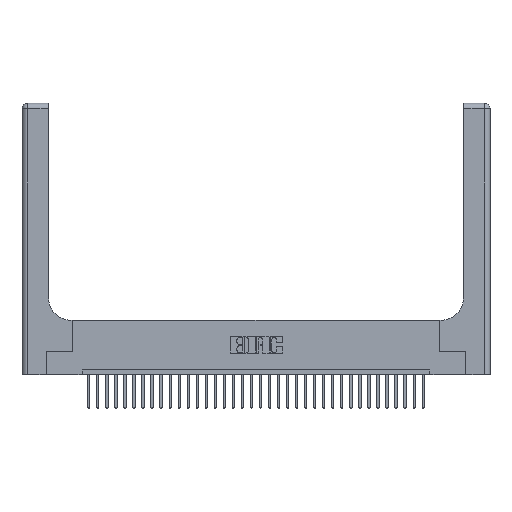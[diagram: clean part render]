
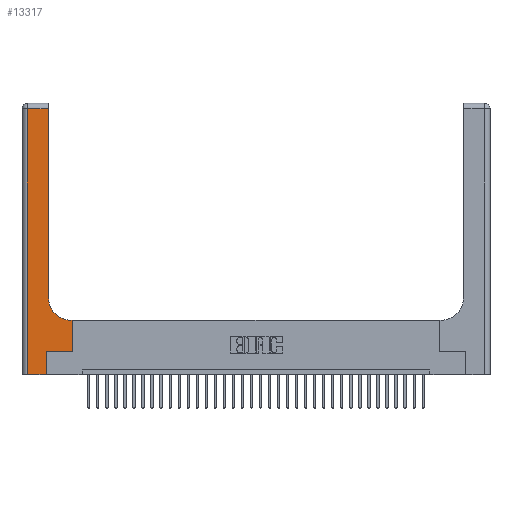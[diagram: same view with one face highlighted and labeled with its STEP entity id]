
A CAD part, top view. The second image highlights one B-rep face of the part: STEP entity #13317.
In plain terms, the highlighted planar face has unit normal (0, 0, 1).
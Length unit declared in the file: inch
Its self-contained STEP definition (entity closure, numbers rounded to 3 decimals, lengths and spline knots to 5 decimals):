
#956 = CARTESIAN_POINT ( 'NONE',  ( 0.5415, 0.6, 0.37 ) ) ;
#1182 = CARTESIAN_POINT ( 'NONE',  ( 0.06, 2.94, 0.37 ) ) ;
#1258 = EDGE_CURVE ( 'NONE', #16805, #28091, #2819, .T. ) ;
#2010 = ORIENTED_EDGE ( 'NONE', *, *, #9235, .T. ) ;
#2102 = CARTESIAN_POINT ( 'NONE',  ( 0.2915, 0.6, 0.37 ) ) ;
#2819 = LINE ( 'NONE', #2102, #31387 ) ;
#2953 = VERTEX_POINT ( 'NONE', #7476 ) ;
#4303 = DIRECTION ( 'NONE',  ( 0., 1., 0. ) ) ;
#4928 = LINE ( 'NONE', #17188, #25613 ) ;
#5272 = LINE ( 'NONE', #17561, #27623 ) ;
#5859 = LINE ( 'NONE', #9953, #17491 ) ;
#6303 = ORIENTED_EDGE ( 'NONE', *, *, #15693, .T. ) ;
#6751 = CARTESIAN_POINT ( 'NONE',  ( 0., 3., 0.37 ) ) ;
#7102 = DIRECTION ( 'NONE',  ( 0., 0., -1. ) ) ;
#7476 = CARTESIAN_POINT ( 'NONE',  ( 0.2915, 0.85, 0.37 ) ) ;
#7660 = CIRCLE ( 'NONE', #20442, 0.25 ) ;
#8048 = VECTOR ( 'NONE', #4303, 39.37008 ) ;
#8104 = EDGE_LOOP ( 'NONE', ( #2010, #31231, #11013, #26593, #19111, #23381, #6303, #32745, #13252 ) ) ;
#8787 = DIRECTION ( 'NONE',  ( 0., -1., 0. ) ) ;
#9042 = VECTOR ( 'NONE', #18088, 39.37008 ) ;
#9235 = EDGE_CURVE ( 'NONE', #2953, #24137, #32086, .T. ) ;
#9812 = LINE ( 'NONE', #19472, #18540 ) ;
#9953 = CARTESIAN_POINT ( 'NONE',  ( 0., 0., 0.37 ) ) ;
#10072 = CARTESIAN_POINT ( 'NONE',  ( 0.269, 0., 0.37 ) ) ;
#10834 = EDGE_CURVE ( 'NONE', #24137, #16845, #30407, .T. ) ;
#11013 = ORIENTED_EDGE ( 'NONE', *, *, #29925, .T. ) ;
#11878 = EDGE_CURVE ( 'NONE', #14102, #22982, #5859, .T. ) ;
#12438 = DIRECTION ( 'NONE',  ( 0., 0., -1. ) ) ;
#13252 = ORIENTED_EDGE ( 'NONE', *, *, #24099, .T. ) ;
#13317 = ADVANCED_FACE ( 'NONE', ( #16155 ), #33529, .F. ) ;
#14102 = VERTEX_POINT ( 'NONE', #27382 ) ;
#14231 = EDGE_CURVE ( 'NONE', #24952, #31144, #4928, .T. ) ;
#15693 = EDGE_CURVE ( 'NONE', #31144, #16805, #5272, .T. ) ;
#16096 = LINE ( 'NONE', #10072, #9042 ) ;
#16155 = FACE_OUTER_BOUND ( 'NONE', #8104, .T. ) ;
#16568 = CARTESIAN_POINT ( 'NONE',  ( 0.2915, 2.94, 0.37 ) ) ;
#16797 = CARTESIAN_POINT ( 'NONE',  ( 0.5585, 0.6, 0.37 ) ) ;
#16805 = VERTEX_POINT ( 'NONE', #16797 ) ;
#16845 = VERTEX_POINT ( 'NONE', #1182 ) ;
#17188 = CARTESIAN_POINT ( 'NONE',  ( 0.269, 0.25, 0.37 ) ) ;
#17491 = VECTOR ( 'NONE', #20611, 39.37008 ) ;
#17561 = CARTESIAN_POINT ( 'NONE',  ( 0.5585, 0.25, 0.37 ) ) ;
#18088 = DIRECTION ( 'NONE',  ( 0., 1., 0. ) ) ;
#18540 = VECTOR ( 'NONE', #8787, 39.37008 ) ;
#18709 = DIRECTION ( 'NONE',  ( -1., 0., 0. ) ) ;
#19111 = ORIENTED_EDGE ( 'NONE', *, *, #26068, .T. ) ;
#19472 = CARTESIAN_POINT ( 'NONE',  ( 0.06, 3., 0.37 ) ) ;
#20410 = DIRECTION ( 'NONE',  ( 1., 0., 0. ) ) ;
#20442 = AXIS2_PLACEMENT_3D ( 'NONE', #22957, #7102, #20410 ) ;
#20611 = DIRECTION ( 'NONE',  ( 1., 0., 0. ) ) ;
#22373 = AXIS2_PLACEMENT_3D ( 'NONE', #6751, #12438, #18709 ) ;
#22646 = DIRECTION ( 'NONE',  ( 0., 1., 0. ) ) ;
#22957 = CARTESIAN_POINT ( 'NONE',  ( 0.5415, 0.85, 0.37 ) ) ;
#22982 = VERTEX_POINT ( 'NONE', #29307 ) ;
#23381 = ORIENTED_EDGE ( 'NONE', *, *, #14231, .T. ) ;
#24099 = EDGE_CURVE ( 'NONE', #28091, #2953, #7660, .T. ) ;
#24137 = VERTEX_POINT ( 'NONE', #16568 ) ;
#24952 = VERTEX_POINT ( 'NONE', #32991 ) ;
#25613 = VECTOR ( 'NONE', #30383, 39.37008 ) ;
#26066 = DIRECTION ( 'NONE',  ( -1., 0., 0. ) ) ;
#26068 = EDGE_CURVE ( 'NONE', #22982, #24952, #16096, .T. ) ;
#26593 = ORIENTED_EDGE ( 'NONE', *, *, #11878, .T. ) ;
#27382 = CARTESIAN_POINT ( 'NONE',  ( 0.06, 0., 0.37 ) ) ;
#27623 = VECTOR ( 'NONE', #22646, 39.37008 ) ;
#28091 = VERTEX_POINT ( 'NONE', #956 ) ;
#29307 = CARTESIAN_POINT ( 'NONE',  ( 0.269, 0., 0.37 ) ) ;
#29671 = DIRECTION ( 'NONE',  ( -1., 0., 0. ) ) ;
#29695 = CARTESIAN_POINT ( 'NONE',  ( 0.5585, 0.25, 0.37 ) ) ;
#29925 = EDGE_CURVE ( 'NONE', #16845, #14102, #9812, .T. ) ;
#30383 = DIRECTION ( 'NONE',  ( 1., 0., 0. ) ) ;
#30407 = LINE ( 'NONE', #32123, #31683 ) ;
#31144 = VERTEX_POINT ( 'NONE', #29695 ) ;
#31231 = ORIENTED_EDGE ( 'NONE', *, *, #10834, .T. ) ;
#31387 = VECTOR ( 'NONE', #26066, 39.37008 ) ;
#31683 = VECTOR ( 'NONE', #29671, 39.37008 ) ;
#32086 = LINE ( 'NONE', #32433, #8048 ) ;
#32123 = CARTESIAN_POINT ( 'NONE',  ( 0., 2.94, 0.37 ) ) ;
#32433 = CARTESIAN_POINT ( 'NONE',  ( 0.2915, 3., 0.37 ) ) ;
#32745 = ORIENTED_EDGE ( 'NONE', *, *, #1258, .T. ) ;
#32991 = CARTESIAN_POINT ( 'NONE',  ( 0.269, 0.25, 0.37 ) ) ;
#33529 = PLANE ( 'NONE',  #22373 ) ;
